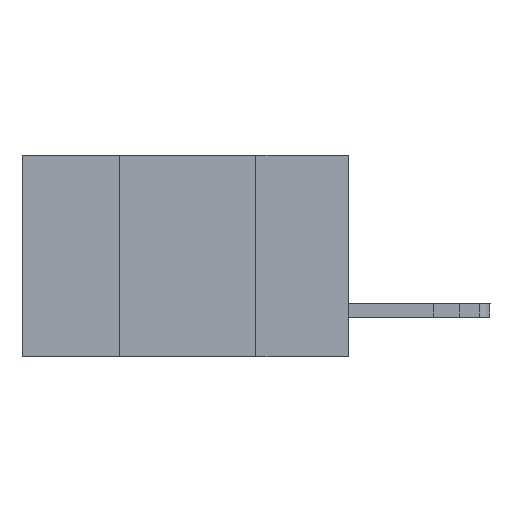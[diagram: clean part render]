
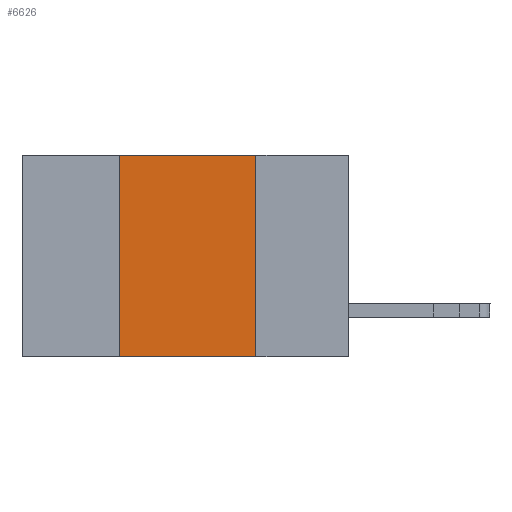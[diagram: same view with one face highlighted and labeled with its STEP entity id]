
A CAD part, left-side view. The second image highlights one B-rep face of the part: STEP entity #6626.
In plain terms, the highlighted planar face has unit normal (-1, 0, 0).
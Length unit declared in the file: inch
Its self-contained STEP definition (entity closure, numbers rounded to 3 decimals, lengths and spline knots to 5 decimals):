
#68 = CARTESIAN_POINT ( 'NONE',  ( 0., 0.42, 0. ) ) ;
#517 = LINE ( 'NONE', #68, #11488 ) ;
#802 = VECTOR ( 'NONE', #6403, 39.37008 ) ;
#806 = PLANE ( 'NONE',  #11048 ) ;
#931 = FACE_OUTER_BOUND ( 'NONE', #9243, .T. ) ;
#1026 = CARTESIAN_POINT ( 'NONE',  ( 0., 0.42, -0.37 ) ) ;
#1049 = LINE ( 'NONE', #10441, #1325 ) ;
#1325 = VECTOR ( 'NONE', #6928, 39.37008 ) ;
#2542 = VERTEX_POINT ( 'NONE', #1026 ) ;
#2628 = ORIENTED_EDGE ( 'NONE', *, *, #7641, .T. ) ;
#2737 = ORIENTED_EDGE ( 'NONE', *, *, #6177, .F. ) ;
#2893 = VERTEX_POINT ( 'NONE', #8201 ) ;
#2911 = DIRECTION ( 'NONE',  ( 0., -1., 0. ) ) ;
#3877 = ORIENTED_EDGE ( 'NONE', *, *, #4785, .F. ) ;
#3882 = CARTESIAN_POINT ( 'NONE',  ( 0., 0.17, -0.37 ) ) ;
#4785 = EDGE_CURVE ( 'NONE', #11445, #2893, #5482, .T. ) ;
#4899 = EDGE_CURVE ( 'NONE', #2542, #11445, #517, .T. ) ;
#5482 = LINE ( 'NONE', #8309, #10360 ) ;
#5673 = ORIENTED_EDGE ( 'NONE', *, *, #4899, .F. ) ;
#6177 = EDGE_CURVE ( 'NONE', #2893, #8118, #11052, .T. ) ;
#6403 = DIRECTION ( 'NONE',  ( 0., 0., -1. ) ) ;
#6419 = DIRECTION ( 'NONE',  ( 0., 0., 1. ) ) ;
#6459 = CARTESIAN_POINT ( 'NONE',  ( 0., 0.42, 0. ) ) ;
#6626 = ADVANCED_FACE ( 'NONE', ( #931 ), #806, .F. ) ;
#6928 = DIRECTION ( 'NONE',  ( 0., -1., 0. ) ) ;
#7312 = DIRECTION ( 'NONE',  ( 1., 0., 0. ) ) ;
#7641 = EDGE_CURVE ( 'NONE', #2542, #8118, #1049, .T. ) ;
#8061 = CARTESIAN_POINT ( 'NONE',  ( 0., 0.6, 0. ) ) ;
#8118 = VERTEX_POINT ( 'NONE', #3882 ) ;
#8201 = CARTESIAN_POINT ( 'NONE',  ( 0., 0.17, 0. ) ) ;
#8309 = CARTESIAN_POINT ( 'NONE',  ( 0., 0.6, 0. ) ) ;
#9124 = DIRECTION ( 'NONE',  ( 0., 0., -1. ) ) ;
#9243 = EDGE_LOOP ( 'NONE', ( #2737, #3877, #5673, #2628 ) ) ;
#9246 = CARTESIAN_POINT ( 'NONE',  ( 0., 0.17, 0. ) ) ;
#10360 = VECTOR ( 'NONE', #2911, 39.37008 ) ;
#10441 = CARTESIAN_POINT ( 'NONE',  ( 0., 0.6, -0.37 ) ) ;
#11048 = AXIS2_PLACEMENT_3D ( 'NONE', #8061, #7312, #9124 ) ;
#11052 = LINE ( 'NONE', #9246, #802 ) ;
#11445 = VERTEX_POINT ( 'NONE', #6459 ) ;
#11488 = VECTOR ( 'NONE', #6419, 39.37008 ) ;
